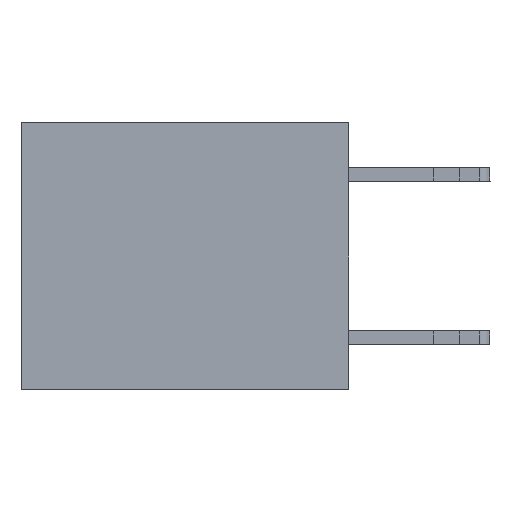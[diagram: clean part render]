
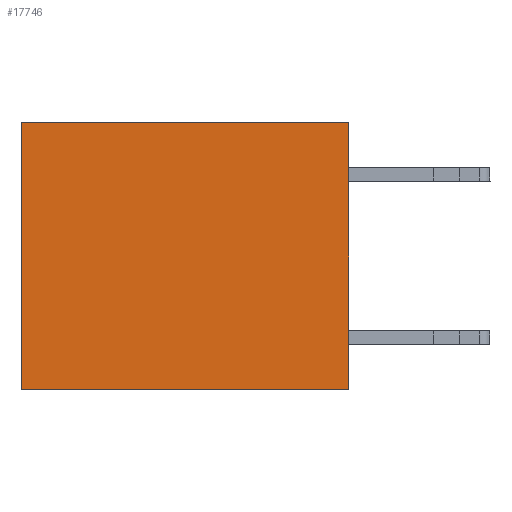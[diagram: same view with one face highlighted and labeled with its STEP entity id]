
A CAD part, left-side view. The second image highlights one B-rep face of the part: STEP entity #17746.
In plain terms, the highlighted planar face has unit normal (-1, 0, 0).
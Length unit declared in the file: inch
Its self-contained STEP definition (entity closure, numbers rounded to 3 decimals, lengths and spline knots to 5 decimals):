
#687 = DIRECTION ( 'NONE',  ( 0., 1., 0. ) ) ;
#2160 = CARTESIAN_POINT ( 'NONE',  ( 0.3165, 0.6, -0.49 ) ) ;
#3581 = DIRECTION ( 'NONE',  ( 0., 1., 0. ) ) ;
#4356 = VERTEX_POINT ( 'NONE', #12607 ) ;
#4614 = LINE ( 'NONE', #16079, #19636 ) ;
#6212 = FACE_OUTER_BOUND ( 'NONE', #8579, .T. ) ;
#6787 = DIRECTION ( 'NONE',  ( 0., 0., -1. ) ) ;
#7333 = AXIS2_PLACEMENT_3D ( 'NONE', #24883, #24613, #6787 ) ;
#7587 = CARTESIAN_POINT ( 'NONE',  ( 0.3165, 0., -0.49 ) ) ;
#7800 = ORIENTED_EDGE ( 'NONE', *, *, #16706, .F. ) ;
#8579 = EDGE_LOOP ( 'NONE', ( #15562, #7800, #27079, #20299 ) ) ;
#10550 = LINE ( 'NONE', #18811, #15093 ) ;
#11291 = PLANE ( 'NONE',  #7333 ) ;
#11295 = CARTESIAN_POINT ( 'NONE',  ( 0.3165, 0., 0. ) ) ;
#12607 = CARTESIAN_POINT ( 'NONE',  ( 0.3165, 0.6, 0. ) ) ;
#14309 = LINE ( 'NONE', #7587, #24704 ) ;
#15093 = VECTOR ( 'NONE', #3581, 39.37008 ) ;
#15562 = ORIENTED_EDGE ( 'NONE', *, *, #19369, .T. ) ;
#16079 = CARTESIAN_POINT ( 'NONE',  ( 0.3165, 0., -0.49 ) ) ;
#16592 = LINE ( 'NONE', #2160, #26959 ) ;
#16706 = EDGE_CURVE ( 'NONE', #19695, #22476, #14309, .T. ) ;
#17746 = ADVANCED_FACE ( 'NONE', ( #6212 ), #11291, .F. ) ;
#18811 = CARTESIAN_POINT ( 'NONE',  ( 0.3165, 0., 0. ) ) ;
#19369 = EDGE_CURVE ( 'NONE', #4356, #22476, #16592, .T. ) ;
#19636 = VECTOR ( 'NONE', #22796, 39.37008 ) ;
#19695 = VERTEX_POINT ( 'NONE', #20689 ) ;
#20299 = ORIENTED_EDGE ( 'NONE', *, *, #23169, .T. ) ;
#20689 = CARTESIAN_POINT ( 'NONE',  ( 0.3165, 0., -0.49 ) ) ;
#22476 = VERTEX_POINT ( 'NONE', #26979 ) ;
#22796 = DIRECTION ( 'NONE',  ( 0., 0., -1. ) ) ;
#23169 = EDGE_CURVE ( 'NONE', #27849, #4356, #10550, .T. ) ;
#24613 = DIRECTION ( 'NONE',  ( 1., 0., 0. ) ) ;
#24639 = DIRECTION ( 'NONE',  ( 0., 0., -1. ) ) ;
#24704 = VECTOR ( 'NONE', #687, 39.37008 ) ;
#24883 = CARTESIAN_POINT ( 'NONE',  ( 0.3165, 0., -0.49 ) ) ;
#26959 = VECTOR ( 'NONE', #24639, 39.37008 ) ;
#26979 = CARTESIAN_POINT ( 'NONE',  ( 0.3165, 0.6, -0.49 ) ) ;
#27079 = ORIENTED_EDGE ( 'NONE', *, *, #27890, .F. ) ;
#27849 = VERTEX_POINT ( 'NONE', #11295 ) ;
#27890 = EDGE_CURVE ( 'NONE', #27849, #19695, #4614, .T. ) ;
